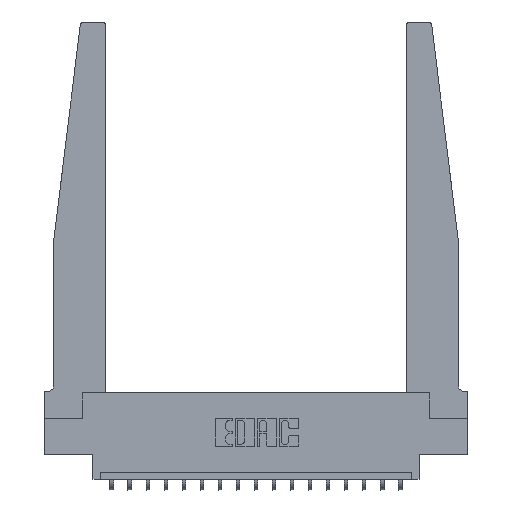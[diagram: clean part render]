
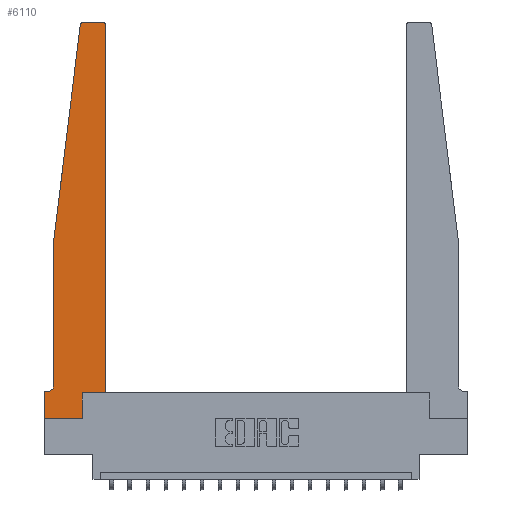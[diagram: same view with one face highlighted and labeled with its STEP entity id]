
A CAD part, top view. The second image highlights one B-rep face of the part: STEP entity #6110.
In plain terms, the highlighted planar face has unit normal (0, 0, 1).
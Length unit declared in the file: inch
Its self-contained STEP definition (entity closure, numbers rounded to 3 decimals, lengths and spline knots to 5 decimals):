
#2 = EDGE_CURVE ( 'NONE', #4160, #288, #18530, .T. ) ;
#288 = VERTEX_POINT ( 'NONE', #9556 ) ;
#328 = VERTEX_POINT ( 'NONE', #15429 ) ;
#589 = DIRECTION ( 'NONE',  ( 1., 0., 0. ) ) ;
#768 = VERTEX_POINT ( 'NONE', #3311 ) ;
#893 = CIRCLE ( 'NONE', #13653, 0.03 ) ;
#1293 = DIRECTION ( 'NONE',  ( 0., 1., 0. ) ) ;
#1314 = AXIS2_PLACEMENT_3D ( 'NONE', #14619, #5859, #16060 ) ;
#1321 = CARTESIAN_POINT ( 'NONE',  ( 0.065, 0.1875, 0.37 ) ) ;
#1526 = FACE_OUTER_BOUND ( 'NONE', #11305, .T. ) ;
#1573 = CARTESIAN_POINT ( 'NONE',  ( 0.24675, 2.72367, 0.37 ) ) ;
#1618 = LINE ( 'NONE', #16918, #9485 ) ;
#1693 = DIRECTION ( 'NONE',  ( 1., 0., 0. ) ) ;
#1940 = VECTOR ( 'NONE', #8222, 39.37008 ) ;
#2127 = LINE ( 'NONE', #9409, #5603 ) ;
#2428 = EDGE_CURVE ( 'NONE', #768, #3715, #5924, .T. ) ;
#2643 = VECTOR ( 'NONE', #5864, 39.37008 ) ;
#2945 = DIRECTION ( 'NONE',  ( 0., 0., -1. ) ) ;
#3311 = CARTESIAN_POINT ( 'NONE',  ( 0., 0.1875, 0.37 ) ) ;
#3469 = DIRECTION ( 'NONE',  ( -1., 0., 0. ) ) ;
#3715 = VERTEX_POINT ( 'NONE', #3888 ) ;
#3782 = CARTESIAN_POINT ( 'NONE',  ( 0.065, 1.25, 0.37 ) ) ;
#3888 = CARTESIAN_POINT ( 'NONE',  ( 0., 0., 0.37 ) ) ;
#3926 = EDGE_CURVE ( 'NONE', #288, #768, #5407, .T. ) ;
#3990 = VERTEX_POINT ( 'NONE', #1573 ) ;
#4160 = VERTEX_POINT ( 'NONE', #12576 ) ;
#4773 = EDGE_CURVE ( 'NONE', #9476, #328, #18148, .T. ) ;
#4924 = EDGE_CURVE ( 'NONE', #3715, #9325, #11642, .T. ) ;
#5037 = EDGE_CURVE ( 'NONE', #10968, #4160, #5863, .T. ) ;
#5347 = DIRECTION ( 'NONE',  ( 0., -1., 0. ) ) ;
#5407 = LINE ( 'NONE', #1321, #8917 ) ;
#5603 = VECTOR ( 'NONE', #9338, 39.37008 ) ;
#5859 = DIRECTION ( 'NONE',  ( 0., 0., 1. ) ) ;
#5863 = LINE ( 'NONE', #15431, #1940 ) ;
#5864 = DIRECTION ( 'NONE',  ( 1., 0., 0. ) ) ;
#5924 = LINE ( 'NONE', #17005, #9423 ) ;
#6110 = ADVANCED_FACE ( 'NONE', ( #1526 ), #9076, .T. ) ;
#6201 = VERTEX_POINT ( 'NONE', #9257 ) ;
#6668 = EDGE_CURVE ( 'NONE', #18003, #6201, #15252, .T. ) ;
#6834 = ORIENTED_EDGE ( 'NONE', *, *, #14918, .T. ) ;
#7165 = ORIENTED_EDGE ( 'NONE', *, *, #6668, .T. ) ;
#7626 = ORIENTED_EDGE ( 'NONE', *, *, #4924, .T. ) ;
#7715 = ORIENTED_EDGE ( 'NONE', *, *, #2, .T. ) ;
#8222 = DIRECTION ( 'NONE',  ( 0., -1., 0. ) ) ;
#8831 = ORIENTED_EDGE ( 'NONE', *, *, #12671, .T. ) ;
#8896 = ORIENTED_EDGE ( 'NONE', *, *, #18824, .T. ) ;
#8917 = VECTOR ( 'NONE', #11758, 39.37008 ) ;
#8928 = CARTESIAN_POINT ( 'NONE',  ( 0.015, 0.2375, 0.37 ) ) ;
#9076 = PLANE ( 'NONE',  #10937 ) ;
#9257 = CARTESIAN_POINT ( 'NONE',  ( 0.395, 2.75, 0.37 ) ) ;
#9325 = VERTEX_POINT ( 'NONE', #17665 ) ;
#9338 = DIRECTION ( 'NONE',  ( -0.122, -0.992, 0. ) ) ;
#9375 = CARTESIAN_POINT ( 'NONE',  ( 0.25, 2.75, 0.37 ) ) ;
#9409 = CARTESIAN_POINT ( 'NONE',  ( 0.065, 1.25, 0.37 ) ) ;
#9420 = CARTESIAN_POINT ( 'NONE',  ( 0.2605, 0.18, 0.37 ) ) ;
#9423 = VECTOR ( 'NONE', #5347, 39.37008 ) ;
#9433 = DIRECTION ( 'NONE',  ( 0., 0., 1. ) ) ;
#9476 = VERTEX_POINT ( 'NONE', #9420 ) ;
#9485 = VECTOR ( 'NONE', #14052, 39.37008 ) ;
#9556 = CARTESIAN_POINT ( 'NONE',  ( 0.015, 0.1875, 0.37 ) ) ;
#10380 = VECTOR ( 'NONE', #3469, 39.37008 ) ;
#10526 = DIRECTION ( 'NONE',  ( 0., 0., 1. ) ) ;
#10734 = AXIS2_PLACEMENT_3D ( 'NONE', #8928, #2945, #17548 ) ;
#10757 = LINE ( 'NONE', #13043, #18409 ) ;
#10877 = EDGE_CURVE ( 'NONE', #14555, #3990, #893, .T. ) ;
#10937 = AXIS2_PLACEMENT_3D ( 'NONE', #13386, #10526, #1693 ) ;
#10968 = VERTEX_POINT ( 'NONE', #3782 ) ;
#11305 = EDGE_LOOP ( 'NONE', ( #18663, #16810, #8896, #16359, #7715, #11986, #12504, #7626, #8831, #13523, #6834, #7165 ) ) ;
#11642 = LINE ( 'NONE', #15123, #15465 ) ;
#11758 = DIRECTION ( 'NONE',  ( -1., 0., 0. ) ) ;
#11986 = ORIENTED_EDGE ( 'NONE', *, *, #3926, .T. ) ;
#12081 = CARTESIAN_POINT ( 'NONE',  ( 0.425, 2.72, 0.37 ) ) ;
#12504 = ORIENTED_EDGE ( 'NONE', *, *, #2428, .T. ) ;
#12576 = CARTESIAN_POINT ( 'NONE',  ( 0.065, 0.2375, 0.37 ) ) ;
#12671 = EDGE_CURVE ( 'NONE', #9325, #9476, #1618, .T. ) ;
#13043 = CARTESIAN_POINT ( 'NONE',  ( 0.425, 0.18, 0.37 ) ) ;
#13125 = EDGE_CURVE ( 'NONE', #6201, #14555, #17572, .T. ) ;
#13386 = CARTESIAN_POINT ( 'NONE',  ( 0., 0.1875, 0.37 ) ) ;
#13523 = ORIENTED_EDGE ( 'NONE', *, *, #4773, .T. ) ;
#13653 = AXIS2_PLACEMENT_3D ( 'NONE', #18051, #9433, #589 ) ;
#14052 = DIRECTION ( 'NONE',  ( 0., 1., 0. ) ) ;
#14555 = VERTEX_POINT ( 'NONE', #16630 ) ;
#14619 = CARTESIAN_POINT ( 'NONE',  ( 0.395, 2.72, 0.37 ) ) ;
#14918 = EDGE_CURVE ( 'NONE', #328, #18003, #10757, .T. ) ;
#15123 = CARTESIAN_POINT ( 'NONE',  ( 0., 0., 0.37 ) ) ;
#15252 = CIRCLE ( 'NONE', #1314, 0.03 ) ;
#15429 = CARTESIAN_POINT ( 'NONE',  ( 0.425, 0.18, 0.37 ) ) ;
#15431 = CARTESIAN_POINT ( 'NONE',  ( 0.065, 1.25, 0.37 ) ) ;
#15465 = VECTOR ( 'NONE', #16562, 39.37008 ) ;
#16060 = DIRECTION ( 'NONE',  ( 1., 0., 0. ) ) ;
#16359 = ORIENTED_EDGE ( 'NONE', *, *, #5037, .T. ) ;
#16562 = DIRECTION ( 'NONE',  ( 1., 0., 0. ) ) ;
#16630 = CARTESIAN_POINT ( 'NONE',  ( 0.27653, 2.75, 0.37 ) ) ;
#16810 = ORIENTED_EDGE ( 'NONE', *, *, #10877, .T. ) ;
#16918 = CARTESIAN_POINT ( 'NONE',  ( 0.2605, 0.18, 0.37 ) ) ;
#17005 = CARTESIAN_POINT ( 'NONE',  ( 0., 0., 0.37 ) ) ;
#17494 = CARTESIAN_POINT ( 'NONE',  ( 0.425, 0.18, 0.37 ) ) ;
#17548 = DIRECTION ( 'NONE',  ( -1., 0., 0. ) ) ;
#17572 = LINE ( 'NONE', #9375, #10380 ) ;
#17665 = CARTESIAN_POINT ( 'NONE',  ( 0.2605, 0., 0.37 ) ) ;
#18003 = VERTEX_POINT ( 'NONE', #12081 ) ;
#18051 = CARTESIAN_POINT ( 'NONE',  ( 0.27653, 2.72, 0.37 ) ) ;
#18148 = LINE ( 'NONE', #17494, #2643 ) ;
#18409 = VECTOR ( 'NONE', #1293, 39.37008 ) ;
#18530 = CIRCLE ( 'NONE', #10734, 0.05 ) ;
#18663 = ORIENTED_EDGE ( 'NONE', *, *, #13125, .T. ) ;
#18824 = EDGE_CURVE ( 'NONE', #3990, #10968, #2127, .T. ) ;
